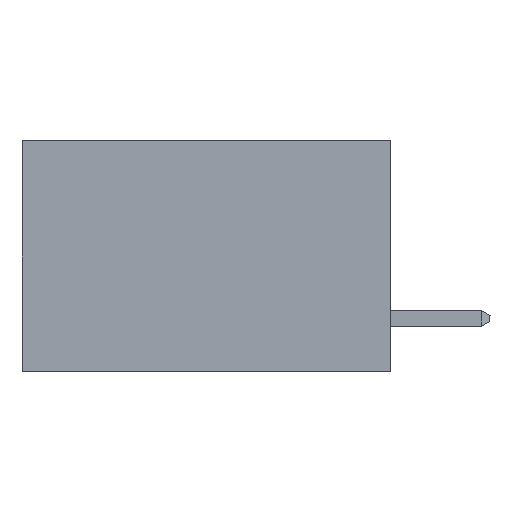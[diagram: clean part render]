
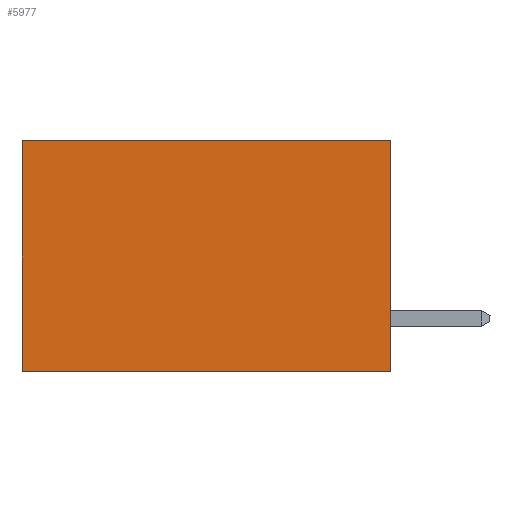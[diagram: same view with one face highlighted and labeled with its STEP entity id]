
A CAD part, left-side view. The second image highlights one B-rep face of the part: STEP entity #5977.
In plain terms, the highlighted planar face has unit normal (-1, 0, 0).
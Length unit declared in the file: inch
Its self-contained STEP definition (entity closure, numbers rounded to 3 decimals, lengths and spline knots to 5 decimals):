
#61 = VECTOR ( 'NONE', #2757, 39.37008 ) ;
#522 = EDGE_LOOP ( 'NONE', ( #2681, #3575, #4494, #5106 ) ) ;
#789 = VECTOR ( 'NONE', #3913, 39.37008 ) ;
#1213 = CARTESIAN_POINT ( 'NONE',  ( 0.277, 0., 0. ) ) ;
#1259 = VECTOR ( 'NONE', #3558, 39.37008 ) ;
#1839 = VERTEX_POINT ( 'NONE', #10373 ) ;
#1962 = VERTEX_POINT ( 'NONE', #9068 ) ;
#2673 = EDGE_CURVE ( 'NONE', #4682, #1839, #11780, .T. ) ;
#2681 = ORIENTED_EDGE ( 'NONE', *, *, #4920, .T. ) ;
#2757 = DIRECTION ( 'NONE',  ( 0., 0., -1. ) ) ;
#2799 = CARTESIAN_POINT ( 'NONE',  ( 0.277, 0., -0.37 ) ) ;
#2803 = LINE ( 'NONE', #2799, #61 ) ;
#3558 = DIRECTION ( 'NONE',  ( 0., 1., 0. ) ) ;
#3575 = ORIENTED_EDGE ( 'NONE', *, *, #6793, .F. ) ;
#3913 = DIRECTION ( 'NONE',  ( 0., 1., 0. ) ) ;
#3924 = CARTESIAN_POINT ( 'NONE',  ( 0.277, 0., -0.37 ) ) ;
#4418 = CARTESIAN_POINT ( 'NONE',  ( 0.277, 0., 0. ) ) ;
#4494 = ORIENTED_EDGE ( 'NONE', *, *, #6829, .F. ) ;
#4682 = VERTEX_POINT ( 'NONE', #1213 ) ;
#4920 = EDGE_CURVE ( 'NONE', #1839, #11945, #9999, .T. ) ;
#5106 = ORIENTED_EDGE ( 'NONE', *, *, #2673, .T. ) ;
#5977 = ADVANCED_FACE ( 'NONE', ( #11611 ), #8323, .F. ) ;
#6793 = EDGE_CURVE ( 'NONE', #1962, #11945, #7240, .T. ) ;
#6829 = EDGE_CURVE ( 'NONE', #4682, #1962, #2803, .T. ) ;
#7240 = LINE ( 'NONE', #3924, #789 ) ;
#8123 = DIRECTION ( 'NONE',  ( 1., 0., 0. ) ) ;
#8186 = DIRECTION ( 'NONE',  ( 0., 0., -1. ) ) ;
#8323 = PLANE ( 'NONE',  #10522 ) ;
#9068 = CARTESIAN_POINT ( 'NONE',  ( 0.277, 0., -0.37 ) ) ;
#9237 = CARTESIAN_POINT ( 'NONE',  ( 0.277, 0., -0.37 ) ) ;
#9423 = DIRECTION ( 'NONE',  ( 0., 0., -1. ) ) ;
#9701 = VECTOR ( 'NONE', #9423, 39.37008 ) ;
#9999 = LINE ( 'NONE', #10904, #9701 ) ;
#10373 = CARTESIAN_POINT ( 'NONE',  ( 0.277, 0.59, 0. ) ) ;
#10522 = AXIS2_PLACEMENT_3D ( 'NONE', #9237, #8123, #8186 ) ;
#10904 = CARTESIAN_POINT ( 'NONE',  ( 0.277, 0.59, -0.37 ) ) ;
#11611 = FACE_OUTER_BOUND ( 'NONE', #522, .T. ) ;
#11780 = LINE ( 'NONE', #4418, #1259 ) ;
#11945 = VERTEX_POINT ( 'NONE', #11956 ) ;
#11956 = CARTESIAN_POINT ( 'NONE',  ( 0.277, 0.59, -0.37 ) ) ;
